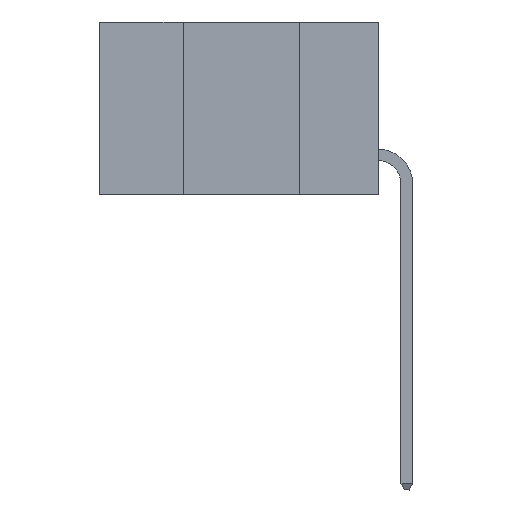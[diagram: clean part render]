
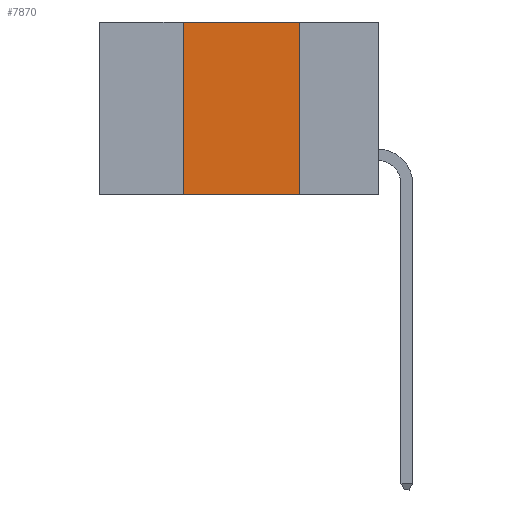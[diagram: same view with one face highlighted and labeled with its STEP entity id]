
A CAD part, left-side view. The second image highlights one B-rep face of the part: STEP entity #7870.
In plain terms, the highlighted planar face has unit normal (-1, 0, 0).
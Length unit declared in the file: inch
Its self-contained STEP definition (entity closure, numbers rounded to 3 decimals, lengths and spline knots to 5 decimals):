
#76 = DIRECTION ( 'NONE',  ( 1., 0., 0. ) ) ;
#763 = PLANE ( 'NONE',  #1180 ) ;
#1180 = AXIS2_PLACEMENT_3D ( 'NONE', #2967, #76, #7747 ) ;
#1292 = VERTEX_POINT ( 'NONE', #2317 ) ;
#1624 = LINE ( 'NONE', #7303, #10285 ) ;
#2096 = EDGE_CURVE ( 'NONE', #11211, #1292, #8263, .T. ) ;
#2317 = CARTESIAN_POINT ( 'NONE',  ( 0., 0.17, -0.37 ) ) ;
#2438 = DIRECTION ( 'NONE',  ( 0., 0., 1. ) ) ;
#2967 = CARTESIAN_POINT ( 'NONE',  ( 0., 0.6, 0. ) ) ;
#3545 = VERTEX_POINT ( 'NONE', #7799 ) ;
#3605 = LINE ( 'NONE', #3784, #11269 ) ;
#3784 = CARTESIAN_POINT ( 'NONE',  ( 0., 0.6, 0. ) ) ;
#3868 = EDGE_LOOP ( 'NONE', ( #11096, #8069, #4764, #9825 ) ) ;
#4080 = CARTESIAN_POINT ( 'NONE',  ( 0., 0.6, -0.37 ) ) ;
#4297 = CARTESIAN_POINT ( 'NONE',  ( 0., 0.42, 0. ) ) ;
#4304 = CARTESIAN_POINT ( 'NONE',  ( 0., 0.17, 0. ) ) ;
#4764 = ORIENTED_EDGE ( 'NONE', *, *, #5002, .F. ) ;
#5002 = EDGE_CURVE ( 'NONE', #3545, #5751, #1624, .T. ) ;
#5489 = VECTOR ( 'NONE', #10428, 39.37008 ) ;
#5751 = VERTEX_POINT ( 'NONE', #4297 ) ;
#5925 = EDGE_CURVE ( 'NONE', #5751, #11211, #3605, .T. ) ;
#6802 = FACE_OUTER_BOUND ( 'NONE', #3868, .T. ) ;
#7303 = CARTESIAN_POINT ( 'NONE',  ( 0., 0.42, -0.37 ) ) ;
#7747 = DIRECTION ( 'NONE',  ( 0., 0., -1. ) ) ;
#7799 = CARTESIAN_POINT ( 'NONE',  ( 0., 0.42, -0.37 ) ) ;
#7870 = ADVANCED_FACE ( 'NONE', ( #6802 ), #763, .F. ) ;
#8055 = EDGE_CURVE ( 'NONE', #3545, #1292, #11681, .T. ) ;
#8069 = ORIENTED_EDGE ( 'NONE', *, *, #5925, .F. ) ;
#8263 = LINE ( 'NONE', #10317, #5489 ) ;
#9040 = VECTOR ( 'NONE', #10916, 39.37008 ) ;
#9825 = ORIENTED_EDGE ( 'NONE', *, *, #8055, .T. ) ;
#10285 = VECTOR ( 'NONE', #2438, 39.37008 ) ;
#10317 = CARTESIAN_POINT ( 'NONE',  ( 0., 0.17, -0.37 ) ) ;
#10428 = DIRECTION ( 'NONE',  ( 0., 0., -1. ) ) ;
#10552 = DIRECTION ( 'NONE',  ( 0., -1., 0. ) ) ;
#10916 = DIRECTION ( 'NONE',  ( 0., -1., 0. ) ) ;
#11096 = ORIENTED_EDGE ( 'NONE', *, *, #2096, .F. ) ;
#11211 = VERTEX_POINT ( 'NONE', #4304 ) ;
#11269 = VECTOR ( 'NONE', #10552, 39.37008 ) ;
#11681 = LINE ( 'NONE', #4080, #9040 ) ;
